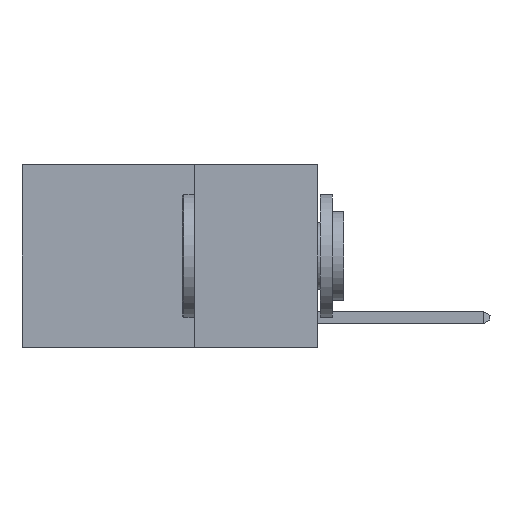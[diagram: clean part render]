
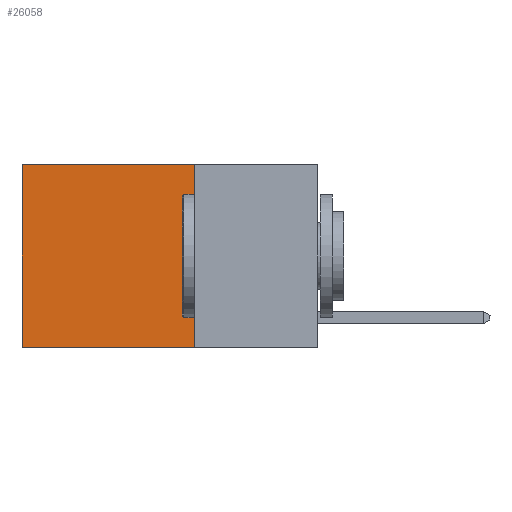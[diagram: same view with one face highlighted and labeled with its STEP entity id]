
A CAD part, left-side view. The second image highlights one B-rep face of the part: STEP entity #26058.
In plain terms, the highlighted planar face has unit normal (-1, 0, 0).
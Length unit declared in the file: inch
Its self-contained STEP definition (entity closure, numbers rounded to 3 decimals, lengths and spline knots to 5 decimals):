
#1019 = EDGE_CURVE ( 'NONE', #5116, #25804, #9472, .T. ) ;
#2230 = VECTOR ( 'NONE', #23636, 39.37008 ) ;
#2926 = VECTOR ( 'NONE', #26521, 39.37008 ) ;
#3743 = CARTESIAN_POINT ( 'NONE',  ( 0.2625, 0.25, 0. ) ) ;
#5116 = VERTEX_POINT ( 'NONE', #3743 ) ;
#5698 = AXIS2_PLACEMENT_3D ( 'NONE', #18024, #24735, #11264 ) ;
#5805 = VECTOR ( 'NONE', #26142, 39.37008 ) ;
#6292 = CARTESIAN_POINT ( 'NONE',  ( 0.2625, 0.25, 0. ) ) ;
#6323 = CARTESIAN_POINT ( 'NONE',  ( 0.2625, 0.25, -0.37 ) ) ;
#6534 = LINE ( 'NONE', #23934, #5805 ) ;
#8286 = LINE ( 'NONE', #10041, #2230 ) ;
#8820 = ORIENTED_EDGE ( 'NONE', *, *, #1019, .T. ) ;
#8994 = PLANE ( 'NONE',  #5698 ) ;
#9472 = LINE ( 'NONE', #12197, #26691 ) ;
#10041 = CARTESIAN_POINT ( 'NONE',  ( 0.2625, 0.25, -0.37 ) ) ;
#10055 = FACE_OUTER_BOUND ( 'NONE', #15792, .T. ) ;
#10487 = VERTEX_POINT ( 'NONE', #6323 ) ;
#11264 = DIRECTION ( 'NONE',  ( 0., 0., -1. ) ) ;
#12009 = CARTESIAN_POINT ( 'NONE',  ( 0.2625, 0.6, 0. ) ) ;
#12197 = CARTESIAN_POINT ( 'NONE',  ( 0.2625, 0.25, 0. ) ) ;
#15792 = EDGE_LOOP ( 'NONE', ( #22378, #21605, #25877, #8820 ) ) ;
#16688 = EDGE_CURVE ( 'NONE', #25804, #20444, #6534, .T. ) ;
#16789 = EDGE_CURVE ( 'NONE', #5116, #10487, #26903, .T. ) ;
#18024 = CARTESIAN_POINT ( 'NONE',  ( 0.2625, 0.25, 0. ) ) ;
#18641 = EDGE_CURVE ( 'NONE', #10487, #20444, #8286, .T. ) ;
#20444 = VERTEX_POINT ( 'NONE', #22956 ) ;
#21605 = ORIENTED_EDGE ( 'NONE', *, *, #18641, .F. ) ;
#22378 = ORIENTED_EDGE ( 'NONE', *, *, #16688, .T. ) ;
#22956 = CARTESIAN_POINT ( 'NONE',  ( 0.2625, 0.6, -0.37 ) ) ;
#23636 = DIRECTION ( 'NONE',  ( 0., 1., 0. ) ) ;
#23934 = CARTESIAN_POINT ( 'NONE',  ( 0.2625, 0.6, 0. ) ) ;
#24735 = DIRECTION ( 'NONE',  ( 1., 0., 0. ) ) ;
#25621 = DIRECTION ( 'NONE',  ( 0., 1., 0. ) ) ;
#25804 = VERTEX_POINT ( 'NONE', #12009 ) ;
#25877 = ORIENTED_EDGE ( 'NONE', *, *, #16789, .F. ) ;
#26058 = ADVANCED_FACE ( 'NONE', ( #10055 ), #8994, .F. ) ;
#26142 = DIRECTION ( 'NONE',  ( 0., 0., -1. ) ) ;
#26521 = DIRECTION ( 'NONE',  ( 0., 0., -1. ) ) ;
#26691 = VECTOR ( 'NONE', #25621, 39.37008 ) ;
#26903 = LINE ( 'NONE', #6292, #2926 ) ;
